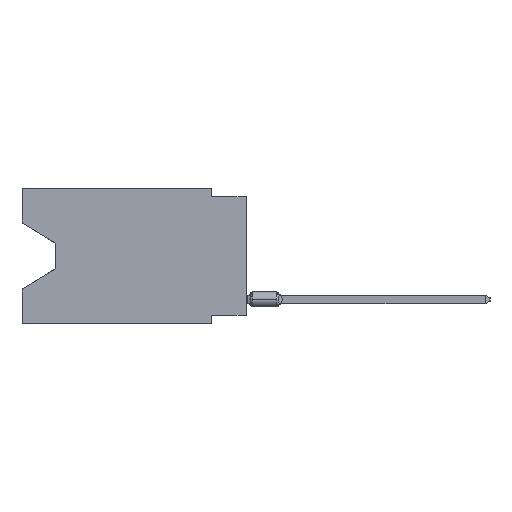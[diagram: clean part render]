
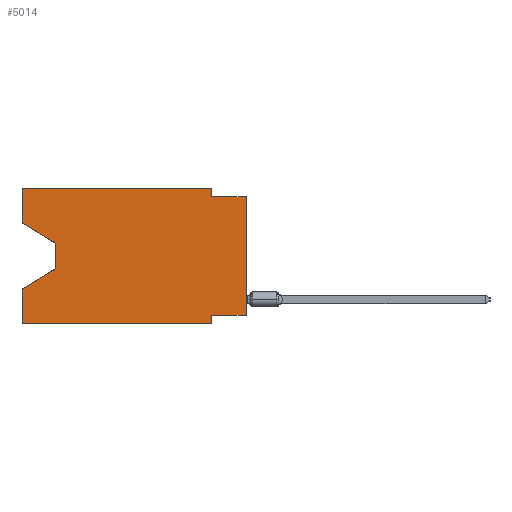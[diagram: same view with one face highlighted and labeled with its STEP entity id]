
A CAD part, left-side view. The second image highlights one B-rep face of the part: STEP entity #5014.
In plain terms, the highlighted planar face has unit normal (-1, 0, 0).
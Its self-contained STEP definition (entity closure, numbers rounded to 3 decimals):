
#329 = EDGE_CURVE ( 'NONE', #7055, #52293, #49628, .T. ) ;
#2443 = ORIENTED_EDGE ( 'NONE', *, *, #14337, .F. ) ;
#4663 = VECTOR ( 'NONE', #43761, 1000. ) ;
#5014 = ADVANCED_FACE ( 'NONE', ( #54643 ), #60990, .F. ) ;
#5645 = LINE ( 'NONE', #49313, #8742 ) ;
#5702 = CARTESIAN_POINT ( 'NONE',  ( 0., 16.383, -9.906 ) ) ;
#5745 = CARTESIAN_POINT ( 'NONE',  ( 0., 13.97, -4.013 ) ) ;
#6568 = DIRECTION ( 'NONE',  ( 1., 0., 0. ) ) ;
#7055 = VERTEX_POINT ( 'NONE', #18439 ) ;
#8355 = CARTESIAN_POINT ( 'NONE',  ( 0., 16.383, -7.36 ) ) ;
#8742 = VECTOR ( 'NONE', #29872, 1000. ) ;
#9307 = VERTEX_POINT ( 'NONE', #29317 ) ;
#11751 = ORIENTED_EDGE ( 'NONE', *, *, #13164, .F. ) ;
#13164 = EDGE_CURVE ( 'NONE', #37420, #74611, #21328, .T. ) ;
#13236 = DIRECTION ( 'NONE',  ( 0., 1., 0. ) ) ;
#14337 = EDGE_CURVE ( 'NONE', #20199, #52293, #5645, .T. ) ;
#15266 = VECTOR ( 'NONE', #27600, 1000. ) ;
#15584 = DIRECTION ( 'NONE',  ( 0., -0.855, -0.519 ) ) ;
#16108 = CARTESIAN_POINT ( 'NONE',  ( 0., 2.54, 0. ) ) ;
#16768 = LINE ( 'NONE', #22335, #76971 ) ;
#17387 = EDGE_CURVE ( 'NONE', #7055, #54247, #43425, .T. ) ;
#17929 = VERTEX_POINT ( 'NONE', #8355 ) ;
#18439 = CARTESIAN_POINT ( 'NONE',  ( 0., 0., -9.271 ) ) ;
#19970 = LINE ( 'NONE', #62113, #48608 ) ;
#20199 = VERTEX_POINT ( 'NONE', #66923 ) ;
#20413 = LINE ( 'NONE', #56214, #36638 ) ;
#20935 = DIRECTION ( 'NONE',  ( 0., -1., 0. ) ) ;
#21328 = LINE ( 'NONE', #45973, #24807 ) ;
#21350 = VERTEX_POINT ( 'NONE', #5745 ) ;
#21727 = DIRECTION ( 'NONE',  ( 0., 0.855, -0.519 ) ) ;
#22134 = CARTESIAN_POINT ( 'NONE',  ( 0., 13.97, -4.013 ) ) ;
#22335 = CARTESIAN_POINT ( 'NONE',  ( 0., 16.383, -2.546 ) ) ;
#23851 = ORIENTED_EDGE ( 'NONE', *, *, #17387, .F. ) ;
#24445 = CARTESIAN_POINT ( 'NONE',  ( 0., 16.383, 0. ) ) ;
#24807 = VECTOR ( 'NONE', #20935, 1000. ) ;
#26021 = DIRECTION ( 'NONE',  ( 0., -1., 0. ) ) ;
#26154 = VECTOR ( 'NONE', #50023, 1000. ) ;
#26363 = LINE ( 'NONE', #68490, #58486 ) ;
#27366 = EDGE_CURVE ( 'NONE', #46611, #37420, #70893, .T. ) ;
#27600 = DIRECTION ( 'NONE',  ( 0., 0., 1. ) ) ;
#27602 = CARTESIAN_POINT ( 'NONE',  ( 0., 2.54, -9.906 ) ) ;
#27603 = ORIENTED_EDGE ( 'NONE', *, *, #72137, .T. ) ;
#27659 = ORIENTED_EDGE ( 'NONE', *, *, #58113, .F. ) ;
#29317 = CARTESIAN_POINT ( 'NONE',  ( 0., 13.97, -5.893 ) ) ;
#29872 = DIRECTION ( 'NONE',  ( 0., -1., 0. ) ) ;
#29921 = EDGE_LOOP ( 'NONE', ( #27603, #50185, #75372, #27659, #54055, #41995, #23851, #36613, #2443, #41121, #11751, #69470 ) ) ;
#31457 = LINE ( 'NONE', #50123, #4663 ) ;
#31881 = VECTOR ( 'NONE', #13236, 1000. ) ;
#35109 = VECTOR ( 'NONE', #46368, 1000. ) ;
#35681 = EDGE_CURVE ( 'NONE', #21350, #9307, #46750, .T. ) ;
#36613 = ORIENTED_EDGE ( 'NONE', *, *, #329, .T. ) ;
#36638 = VECTOR ( 'NONE', #26021, 1000. ) ;
#37420 = VERTEX_POINT ( 'NONE', #70780 ) ;
#37881 = AXIS2_PLACEMENT_3D ( 'NONE', #24445, #6568, #48671 ) ;
#38686 = DIRECTION ( 'NONE',  ( 0., 0., -1. ) ) ;
#39912 = CARTESIAN_POINT ( 'NONE',  ( 0., 16.383, 0. ) ) ;
#40031 = VERTEX_POINT ( 'NONE', #27602 ) ;
#40261 = EDGE_CURVE ( 'NONE', #54247, #40031, #19970, .T. ) ;
#41121 = ORIENTED_EDGE ( 'NONE', *, *, #47530, .F. ) ;
#41995 = ORIENTED_EDGE ( 'NONE', *, *, #40261, .F. ) ;
#43270 = CARTESIAN_POINT ( 'NONE',  ( 0., 0., 0. ) ) ;
#43425 = LINE ( 'NONE', #60928, #31881 ) ;
#43761 = DIRECTION ( 'NONE',  ( 0., 0., 1. ) ) ;
#45973 = CARTESIAN_POINT ( 'NONE',  ( 0., 16.383, 0. ) ) ;
#46368 = DIRECTION ( 'NONE',  ( 0., 0., -1. ) ) ;
#46611 = VERTEX_POINT ( 'NONE', #72695 ) ;
#46750 = LINE ( 'NONE', #22134, #35109 ) ;
#47530 = EDGE_CURVE ( 'NONE', #74611, #20199, #26363, .T. ) ;
#48608 = VECTOR ( 'NONE', #68452, 1000. ) ;
#48671 = DIRECTION ( 'NONE',  ( 0., 0., -1. ) ) ;
#49313 = CARTESIAN_POINT ( 'NONE',  ( 0., 0., -0.635 ) ) ;
#49628 = LINE ( 'NONE', #43270, #26154 ) ;
#50023 = DIRECTION ( 'NONE',  ( 0., 0., 1. ) ) ;
#50123 = CARTESIAN_POINT ( 'NONE',  ( 0., 16.383, 0. ) ) ;
#50185 = ORIENTED_EDGE ( 'NONE', *, *, #35681, .T. ) ;
#52293 = VERTEX_POINT ( 'NONE', #60436 ) ;
#54055 = ORIENTED_EDGE ( 'NONE', *, *, #62516, .T. ) ;
#54135 = EDGE_CURVE ( 'NONE', #9307, #17929, #75751, .T. ) ;
#54247 = VERTEX_POINT ( 'NONE', #78114 ) ;
#54643 = FACE_OUTER_BOUND ( 'NONE', #29921, .T. ) ;
#56214 = CARTESIAN_POINT ( 'NONE',  ( 0., 16.383, -9.906 ) ) ;
#58113 = EDGE_CURVE ( 'NONE', #61593, #17929, #31457, .T. ) ;
#58486 = VECTOR ( 'NONE', #38686, 1000. ) ;
#60436 = CARTESIAN_POINT ( 'NONE',  ( 0., 0., -0.635 ) ) ;
#60928 = CARTESIAN_POINT ( 'NONE',  ( 0., 0., -9.271 ) ) ;
#60990 = PLANE ( 'NONE',  #37881 ) ;
#61320 = VECTOR ( 'NONE', #21727, 1000. ) ;
#61593 = VERTEX_POINT ( 'NONE', #5702 ) ;
#62113 = CARTESIAN_POINT ( 'NONE',  ( 0., 2.54, -9.906 ) ) ;
#62516 = EDGE_CURVE ( 'NONE', #61593, #40031, #20413, .T. ) ;
#63457 = CARTESIAN_POINT ( 'NONE',  ( 0., 13.97, -5.893 ) ) ;
#66923 = CARTESIAN_POINT ( 'NONE',  ( 0., 2.54, -0.635 ) ) ;
#68452 = DIRECTION ( 'NONE',  ( 0., 0., -1. ) ) ;
#68490 = CARTESIAN_POINT ( 'NONE',  ( 0., 2.54, 0. ) ) ;
#69470 = ORIENTED_EDGE ( 'NONE', *, *, #27366, .F. ) ;
#70780 = CARTESIAN_POINT ( 'NONE',  ( 0., 16.383, 0. ) ) ;
#70893 = LINE ( 'NONE', #39912, #15266 ) ;
#72137 = EDGE_CURVE ( 'NONE', #46611, #21350, #16768, .T. ) ;
#72695 = CARTESIAN_POINT ( 'NONE',  ( 0., 16.383, -2.546 ) ) ;
#74611 = VERTEX_POINT ( 'NONE', #16108 ) ;
#75372 = ORIENTED_EDGE ( 'NONE', *, *, #54135, .T. ) ;
#75751 = LINE ( 'NONE', #63457, #61320 ) ;
#76971 = VECTOR ( 'NONE', #15584, 1000. ) ;
#78114 = CARTESIAN_POINT ( 'NONE',  ( 0., 2.54, -9.271 ) ) ;
